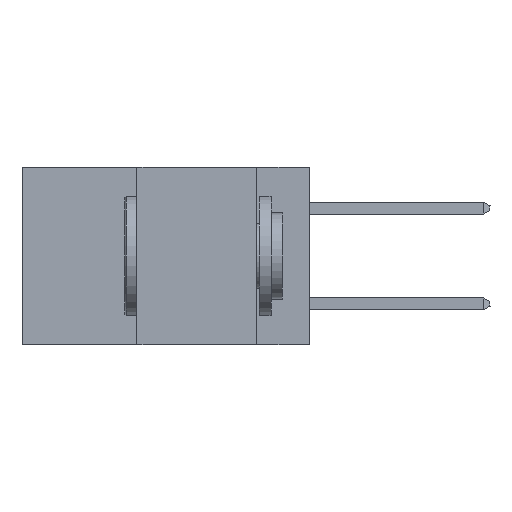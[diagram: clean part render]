
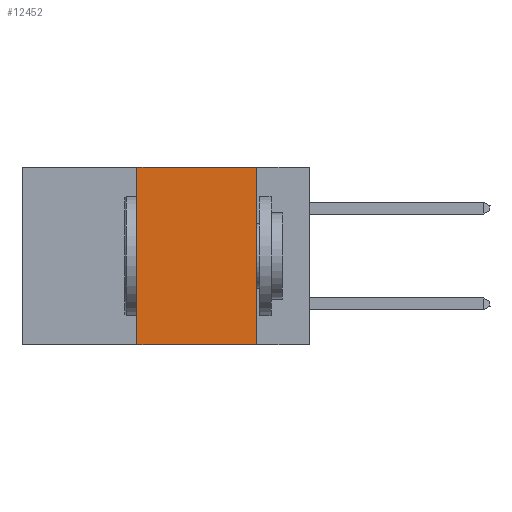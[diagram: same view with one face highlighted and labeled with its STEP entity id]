
A CAD part, left-side view. The second image highlights one B-rep face of the part: STEP entity #12452.
In plain terms, the highlighted planar face has unit normal (-1, 0, 0).
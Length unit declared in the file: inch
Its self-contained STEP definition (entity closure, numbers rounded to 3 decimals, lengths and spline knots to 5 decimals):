
#946 = CARTESIAN_POINT ( 'NONE',  ( 0., 0.11, 0. ) ) ;
#1062 = CARTESIAN_POINT ( 'NONE',  ( 0., 0.6, 0. ) ) ;
#2049 = DIRECTION ( 'NONE',  ( 1., 0., 0. ) ) ;
#2679 = LINE ( 'NONE', #946, #31125 ) ;
#2680 = CARTESIAN_POINT ( 'NONE',  ( 0., 0.11, -0.37 ) ) ;
#3013 = CARTESIAN_POINT ( 'NONE',  ( 0., 0.6, -0.37 ) ) ;
#3139 = LINE ( 'NONE', #1062, #24721 ) ;
#3530 = EDGE_CURVE ( 'NONE', #25751, #20722, #4859, .T. ) ;
#4215 = VECTOR ( 'NONE', #19275, 39.37008 ) ;
#4322 = CARTESIAN_POINT ( 'NONE',  ( 0., 0.36, 0. ) ) ;
#4859 = LINE ( 'NONE', #4322, #21619 ) ;
#5895 = ORIENTED_EDGE ( 'NONE', *, *, #30609, .F. ) ;
#6920 = EDGE_LOOP ( 'NONE', ( #7225, #5895, #31411, #24497 ) ) ;
#7225 = ORIENTED_EDGE ( 'NONE', *, *, #24888, .F. ) ;
#8297 = VERTEX_POINT ( 'NONE', #30965 ) ;
#8756 = FACE_OUTER_BOUND ( 'NONE', #6920, .T. ) ;
#11549 = CARTESIAN_POINT ( 'NONE',  ( 0., 0.6, 0. ) ) ;
#12452 = ADVANCED_FACE ( 'NONE', ( #8756 ), #25684, .F. ) ;
#14920 = DIRECTION ( 'NONE',  ( 0., -1., 0. ) ) ;
#15306 = DIRECTION ( 'NONE',  ( 0., 0., -1. ) ) ;
#19275 = DIRECTION ( 'NONE',  ( 0., -1., 0. ) ) ;
#20722 = VERTEX_POINT ( 'NONE', #24934 ) ;
#21619 = VECTOR ( 'NONE', #34461, 39.37008 ) ;
#22387 = DIRECTION ( 'NONE',  ( 0., 0., -1. ) ) ;
#24497 = ORIENTED_EDGE ( 'NONE', *, *, #33712, .T. ) ;
#24721 = VECTOR ( 'NONE', #14920, 39.37008 ) ;
#24888 = EDGE_CURVE ( 'NONE', #8297, #26080, #2679, .T. ) ;
#24934 = CARTESIAN_POINT ( 'NONE',  ( 0., 0.36, 0. ) ) ;
#25684 = PLANE ( 'NONE',  #32943 ) ;
#25751 = VERTEX_POINT ( 'NONE', #31995 ) ;
#26080 = VERTEX_POINT ( 'NONE', #2680 ) ;
#30609 = EDGE_CURVE ( 'NONE', #20722, #8297, #3139, .T. ) ;
#30965 = CARTESIAN_POINT ( 'NONE',  ( 0., 0.11, 0. ) ) ;
#31125 = VECTOR ( 'NONE', #22387, 39.37008 ) ;
#31411 = ORIENTED_EDGE ( 'NONE', *, *, #3530, .F. ) ;
#31995 = CARTESIAN_POINT ( 'NONE',  ( 0., 0.36, -0.37 ) ) ;
#32943 = AXIS2_PLACEMENT_3D ( 'NONE', #11549, #2049, #15306 ) ;
#33712 = EDGE_CURVE ( 'NONE', #25751, #26080, #35284, .T. ) ;
#34461 = DIRECTION ( 'NONE',  ( 0., 0., 1. ) ) ;
#35284 = LINE ( 'NONE', #3013, #4215 ) ;
